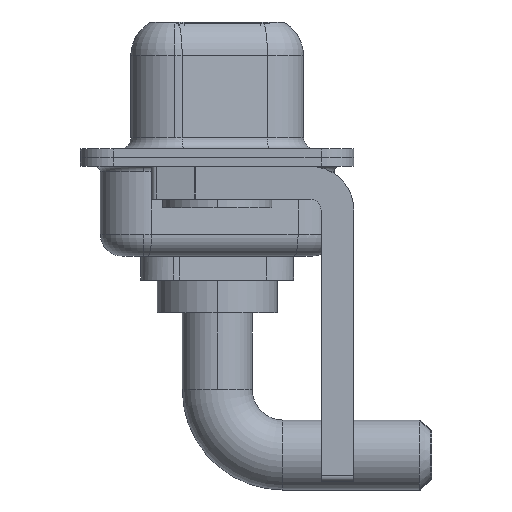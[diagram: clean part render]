
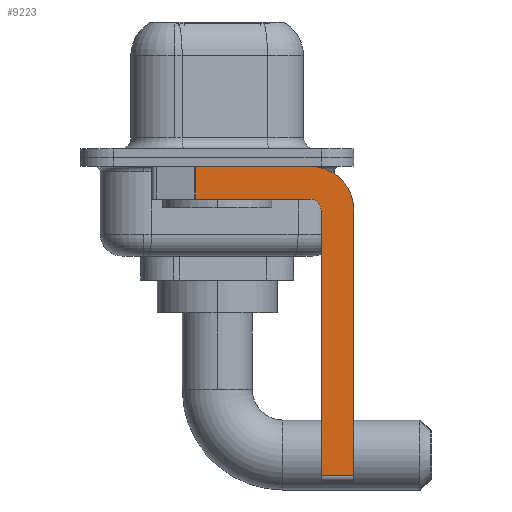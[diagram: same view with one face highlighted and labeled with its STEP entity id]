
A CAD part, left-side view. The second image highlights one B-rep face of the part: STEP entity #9223.
In plain terms, the highlighted planar face has unit normal (-1, 0, 0).
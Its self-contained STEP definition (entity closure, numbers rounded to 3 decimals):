
#119 = ORIENTED_EDGE ( 'NONE', *, *, #2018, .T. ) ;
#984 = CARTESIAN_POINT ( 'NONE',  ( -2.9, -4.25, -14.55 ) ) ;
#1011 = LINE ( 'NONE', #5463, #9777 ) ;
#1305 = CARTESIAN_POINT ( 'NONE',  ( -2.9, -6.25, -2.4 ) ) ;
#1310 = VERTEX_POINT ( 'NONE', #1305 ) ;
#1880 = CARTESIAN_POINT ( 'NONE',  ( -2.9, -6.25, -14.55 ) ) ;
#2018 = EDGE_CURVE ( 'NONE', #10239, #10636, #10169, .T. ) ;
#2028 = VERTEX_POINT ( 'NONE', #6734 ) ;
#2252 = VECTOR ( 'NONE', #10659, 1000. ) ;
#2314 = CARTESIAN_POINT ( 'NONE',  ( -2.9, -6.25, -2.4 ) ) ;
#2402 = DIRECTION ( 'NONE',  ( 0., 0., -1. ) ) ;
#2948 = LINE ( 'NONE', #11858, #4479 ) ;
#3211 = ORIENTED_EDGE ( 'NONE', *, *, #11580, .F. ) ;
#3340 = DIRECTION ( 'NONE',  ( 0., -1., 0. ) ) ;
#3447 = VECTOR ( 'NONE', #3499, 1000. ) ;
#3499 = DIRECTION ( 'NONE',  ( 0., 0., -1. ) ) ;
#3601 = ORIENTED_EDGE ( 'NONE', *, *, #5612, .F. ) ;
#3732 = CARTESIAN_POINT ( 'NONE',  ( -2.9, -4.25, -0.4 ) ) ;
#3760 = CARTESIAN_POINT ( 'NONE',  ( -2.9, 0.978, -1.9 ) ) ;
#4115 = EDGE_CURVE ( 'NONE', #2028, #13461, #11395, .T. ) ;
#4229 = AXIS2_PLACEMENT_3D ( 'NONE', #6730, #14540, #4379 ) ;
#4246 = EDGE_CURVE ( 'NONE', #10239, #11595, #10590, .T. ) ;
#4379 = DIRECTION ( 'NONE',  ( 0., 0., 1. ) ) ;
#4479 = VECTOR ( 'NONE', #7455, 1000. ) ;
#4494 = ORIENTED_EDGE ( 'NONE', *, *, #7382, .F. ) ;
#4877 = DIRECTION ( 'NONE',  ( 0., 0., -1. ) ) ;
#5463 = CARTESIAN_POINT ( 'NONE',  ( -2.9, 3., -0.4 ) ) ;
#5554 = PLANE ( 'NONE',  #11065 ) ;
#5597 = CARTESIAN_POINT ( 'NONE',  ( -2.9, -4.75, -2.4 ) ) ;
#5612 = EDGE_CURVE ( 'NONE', #1310, #10636, #5866, .T. ) ;
#5630 = CARTESIAN_POINT ( 'NONE',  ( -2.9, -4.25, -2.4 ) ) ;
#5866 = LINE ( 'NONE', #2314, #3447 ) ;
#6362 = CIRCLE ( 'NONE', #4229, 0.5 ) ;
#6730 = CARTESIAN_POINT ( 'NONE',  ( -2.9, -4.25, -2.4 ) ) ;
#6734 = CARTESIAN_POINT ( 'NONE',  ( -2.9, 0.978, -0.4 ) ) ;
#6740 = CIRCLE ( 'NONE', #7905, 2. ) ;
#6919 = VECTOR ( 'NONE', #3340, 1000. ) ;
#7382 = EDGE_CURVE ( 'NONE', #11595, #11545, #6362, .T. ) ;
#7443 = CARTESIAN_POINT ( 'NONE',  ( -2.9, -4.75, -14.8 ) ) ;
#7455 = DIRECTION ( 'NONE',  ( 0., 1., 0. ) ) ;
#7581 = CARTESIAN_POINT ( 'NONE',  ( -2.9, -4.75, -14.55 ) ) ;
#7609 = FACE_OUTER_BOUND ( 'NONE', #10296, .T. ) ;
#7698 = EDGE_CURVE ( 'NONE', #11545, #13461, #2948, .T. ) ;
#7792 = DIRECTION ( 'NONE',  ( 0., -1., 0. ) ) ;
#7845 = ORIENTED_EDGE ( 'NONE', *, *, #7698, .F. ) ;
#7905 = AXIS2_PLACEMENT_3D ( 'NONE', #11301, #10200, #2402 ) ;
#8881 = CARTESIAN_POINT ( 'NONE',  ( -2.9, -4.25, -1.9 ) ) ;
#8905 = DIRECTION ( 'NONE',  ( 0., 0., -1. ) ) ;
#9223 = ADVANCED_FACE ( 'NONE', ( #7609 ), #5554, .F. ) ;
#9777 = VECTOR ( 'NONE', #7792, 1000. ) ;
#10169 = LINE ( 'NONE', #984, #6919 ) ;
#10200 = DIRECTION ( 'NONE',  ( 1., 0., 0. ) ) ;
#10239 = VERTEX_POINT ( 'NONE', #7581 ) ;
#10296 = EDGE_LOOP ( 'NONE', ( #3211, #11440, #7845, #4494, #11178, #119, #3601, #13731 ) ) ;
#10421 = VERTEX_POINT ( 'NONE', #3732 ) ;
#10590 = LINE ( 'NONE', #7443, #2252 ) ;
#10636 = VERTEX_POINT ( 'NONE', #1880 ) ;
#10659 = DIRECTION ( 'NONE',  ( 0., 0., 1. ) ) ;
#11065 = AXIS2_PLACEMENT_3D ( 'NONE', #5630, #14528, #8905 ) ;
#11178 = ORIENTED_EDGE ( 'NONE', *, *, #4246, .F. ) ;
#11301 = CARTESIAN_POINT ( 'NONE',  ( -2.9, -4.25, -2.4 ) ) ;
#11395 = LINE ( 'NONE', #3760, #12137 ) ;
#11440 = ORIENTED_EDGE ( 'NONE', *, *, #4115, .T. ) ;
#11545 = VERTEX_POINT ( 'NONE', #8881 ) ;
#11580 = EDGE_CURVE ( 'NONE', #2028, #10421, #1011, .T. ) ;
#11595 = VERTEX_POINT ( 'NONE', #5597 ) ;
#11706 = EDGE_CURVE ( 'NONE', #10421, #1310, #6740, .T. ) ;
#11746 = CARTESIAN_POINT ( 'NONE',  ( -2.9, 0.978, -1.9 ) ) ;
#11858 = CARTESIAN_POINT ( 'NONE',  ( -2.9, -4.25, -1.9 ) ) ;
#12137 = VECTOR ( 'NONE', #4877, 1000. ) ;
#13461 = VERTEX_POINT ( 'NONE', #11746 ) ;
#13731 = ORIENTED_EDGE ( 'NONE', *, *, #11706, .F. ) ;
#14528 = DIRECTION ( 'NONE',  ( 1., 0., 0. ) ) ;
#14540 = DIRECTION ( 'NONE',  ( -1., 0., 0. ) ) ;
